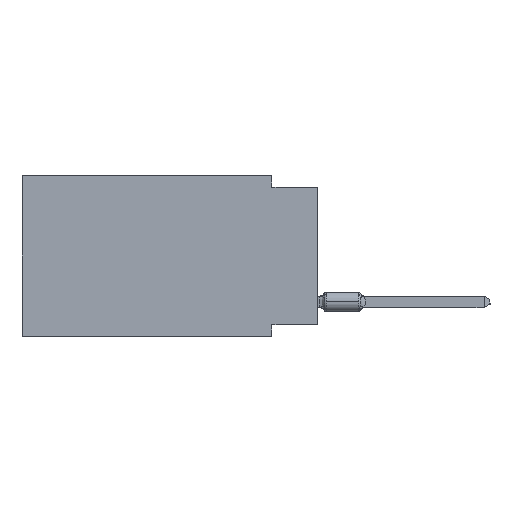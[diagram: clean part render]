
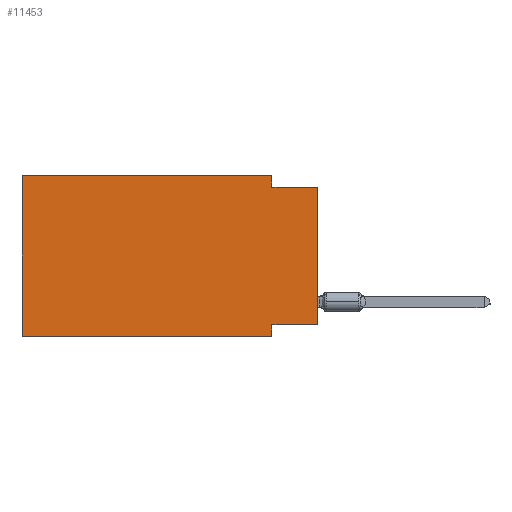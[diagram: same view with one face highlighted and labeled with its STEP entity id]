
A CAD part, left-side view. The second image highlights one B-rep face of the part: STEP entity #11453.
In plain terms, the highlighted planar face has unit normal (-1, 0, 0).
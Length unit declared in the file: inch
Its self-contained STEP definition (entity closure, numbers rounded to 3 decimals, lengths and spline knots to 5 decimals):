
#4 = CARTESIAN_POINT ( 'NONE',  ( 0., 0.645, 0. ) ) ;
#285 = CARTESIAN_POINT ( 'NONE',  ( 0., 0.1, -0.325 ) ) ;
#863 = LINE ( 'NONE', #47172, #30630 ) ;
#1755 = EDGE_CURVE ( 'NONE', #44759, #43312, #10892, .T. ) ;
#2203 = ORIENTED_EDGE ( 'NONE', *, *, #38276, .F. ) ;
#2555 = CARTESIAN_POINT ( 'NONE',  ( 0., 0.645, -0.35 ) ) ;
#3417 = ORIENTED_EDGE ( 'NONE', *, *, #33364, .F. ) ;
#3466 = CARTESIAN_POINT ( 'NONE',  ( 0., 0.1, -0.35 ) ) ;
#3854 = DIRECTION ( 'NONE',  ( 0., 0., -1. ) ) ;
#4821 = CARTESIAN_POINT ( 'NONE',  ( 0., 0., -0.325 ) ) ;
#4832 = VERTEX_POINT ( 'NONE', #3466 ) ;
#5181 = LINE ( 'NONE', #6970, #32973 ) ;
#5399 = CARTESIAN_POINT ( 'NONE',  ( 0., 0.1, 0. ) ) ;
#5943 = CARTESIAN_POINT ( 'NONE',  ( 0., 0., -0.025 ) ) ;
#6970 = CARTESIAN_POINT ( 'NONE',  ( 0., 0.645, 0. ) ) ;
#8521 = ORIENTED_EDGE ( 'NONE', *, *, #24103, .F. ) ;
#9788 = ORIENTED_EDGE ( 'NONE', *, *, #22919, .F. ) ;
#10303 = DIRECTION ( 'NONE',  ( 0., -1., 0. ) ) ;
#10892 = LINE ( 'NONE', #38779, #43853 ) ;
#11453 = ADVANCED_FACE ( 'NONE', ( #16111 ), #31467, .F. ) ;
#12281 = LINE ( 'NONE', #42728, #26623 ) ;
#12574 = ORIENTED_EDGE ( 'NONE', *, *, #38821, .T. ) ;
#12745 = DIRECTION ( 'NONE',  ( 0., 1., 0. ) ) ;
#14320 = DIRECTION ( 'NONE',  ( 0., -1., 0. ) ) ;
#14406 = CARTESIAN_POINT ( 'NONE',  ( 0., 0.645, -0.35 ) ) ;
#14433 = EDGE_CURVE ( 'NONE', #18774, #31550, #12281, .T. ) ;
#15353 = DIRECTION ( 'NONE',  ( 1., 0., 0. ) ) ;
#16111 = FACE_OUTER_BOUND ( 'NONE', #40664, .T. ) ;
#16465 = DIRECTION ( 'NONE',  ( 0., -1., 0. ) ) ;
#17884 = ORIENTED_EDGE ( 'NONE', *, *, #14433, .F. ) ;
#18490 = ORIENTED_EDGE ( 'NONE', *, *, #38998, .F. ) ;
#18774 = VERTEX_POINT ( 'NONE', #14406 ) ;
#22018 = LINE ( 'NONE', #2555, #46088 ) ;
#22919 = EDGE_CURVE ( 'NONE', #45804, #38881, #32023, .T. ) ;
#24103 = EDGE_CURVE ( 'NONE', #38881, #43312, #863, .T. ) ;
#26623 = VECTOR ( 'NONE', #43235, 39.37008 ) ;
#30603 = DIRECTION ( 'NONE',  ( 0., 0., 1. ) ) ;
#30630 = VECTOR ( 'NONE', #16465, 39.37008 ) ;
#30992 = CARTESIAN_POINT ( 'NONE',  ( 0., 0.1, 0. ) ) ;
#31467 = PLANE ( 'NONE',  #46701 ) ;
#31550 = VERTEX_POINT ( 'NONE', #48544 ) ;
#31615 = LINE ( 'NONE', #35196, #40821 ) ;
#32023 = LINE ( 'NONE', #5399, #41281 ) ;
#32973 = VECTOR ( 'NONE', #10303, 39.37008 ) ;
#33364 = EDGE_CURVE ( 'NONE', #48362, #4832, #31615, .T. ) ;
#34946 = DIRECTION ( 'NONE',  ( 0., 0., -1. ) ) ;
#35196 = CARTESIAN_POINT ( 'NONE',  ( 0., 0.1, -0.35 ) ) ;
#38210 = ORIENTED_EDGE ( 'NONE', *, *, #1755, .T. ) ;
#38276 = EDGE_CURVE ( 'NONE', #31550, #45804, #5181, .T. ) ;
#38779 = CARTESIAN_POINT ( 'NONE',  ( 0., 0., 0. ) ) ;
#38821 = EDGE_CURVE ( 'NONE', #18774, #4832, #22018, .T. ) ;
#38881 = VERTEX_POINT ( 'NONE', #39356 ) ;
#38998 = EDGE_CURVE ( 'NONE', #44759, #48362, #39861, .T. ) ;
#39356 = CARTESIAN_POINT ( 'NONE',  ( 0., 0.1, -0.025 ) ) ;
#39861 = LINE ( 'NONE', #4821, #45290 ) ;
#40664 = EDGE_LOOP ( 'NONE', ( #38210, #8521, #9788, #2203, #17884, #12574, #3417, #18490 ) ) ;
#40821 = VECTOR ( 'NONE', #34946, 39.37008 ) ;
#41281 = VECTOR ( 'NONE', #43520, 39.37008 ) ;
#42728 = CARTESIAN_POINT ( 'NONE',  ( 0., 0.645, 0. ) ) ;
#43235 = DIRECTION ( 'NONE',  ( 0., 0., 1. ) ) ;
#43312 = VERTEX_POINT ( 'NONE', #5943 ) ;
#43520 = DIRECTION ( 'NONE',  ( 0., 0., -1. ) ) ;
#43853 = VECTOR ( 'NONE', #30603, 39.37008 ) ;
#44759 = VERTEX_POINT ( 'NONE', #49132 ) ;
#45290 = VECTOR ( 'NONE', #12745, 39.37008 ) ;
#45804 = VERTEX_POINT ( 'NONE', #30992 ) ;
#46088 = VECTOR ( 'NONE', #14320, 39.37008 ) ;
#46701 = AXIS2_PLACEMENT_3D ( 'NONE', #4, #15353, #3854 ) ;
#47172 = CARTESIAN_POINT ( 'NONE',  ( 0., 0., -0.025 ) ) ;
#48362 = VERTEX_POINT ( 'NONE', #285 ) ;
#48544 = CARTESIAN_POINT ( 'NONE',  ( 0., 0.645, 0. ) ) ;
#49132 = CARTESIAN_POINT ( 'NONE',  ( 0., 0., -0.325 ) ) ;
